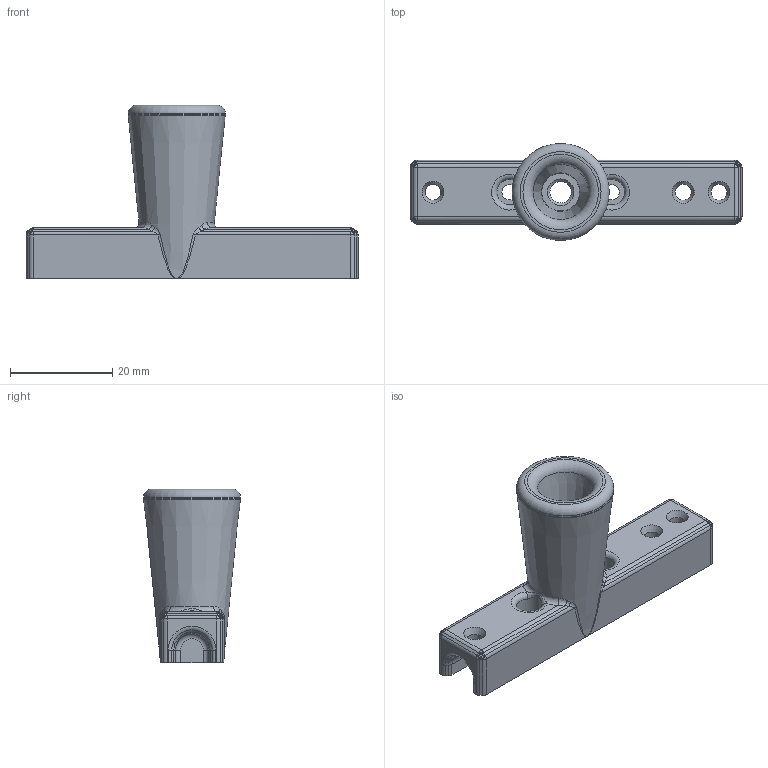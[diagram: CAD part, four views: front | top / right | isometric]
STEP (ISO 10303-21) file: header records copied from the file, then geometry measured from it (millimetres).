
FILE_DESCRIPTION(/* description */ (''),/* implementation_level */ '2;1');
FILE_NAME(/* name */ 'ARK Chargin'' Handle/UnfancyHandle/UnfawncyHandle.step',/* time_stamp */ '2022-02-03T00:25:49-07:00',/* author */ (''),/* organization */ (''),/* preprocessor_version */ 'ST-DEVELOPER v18.1',/* originating_system */ 'Autodesk Translation Framework v10.13.0.1454',/* authorisation */ '');
FILE_SCHEMA (('AUTOMOTIVE_DESIGN { 1 0 10303 214 3 1 1 }'));
Length unit declared in the file: millimetre
Products named in the file (1): UnfawncyHandle
Bounding box: 65 x 19 x 34 mm (x, y, z)
Volume: 10966.7 mm3; surface area: 5623.9 mm2
Topology: 1 solids, 1 shells, 175 faces, 398 edges, 222 vertices
Faces by surface type: cylinder 61, plane 45, sphere 24, bspline 22, cone 12, torus 11
Full cylindrical faces by diameter (mm): 3 x2, 3.1 x3, 4.2 x1, 5 x2, 7.4 x1, 19 x1
Entity records: 5592 total; most frequent: CARTESIAN_POINT 1678, DIRECTION 839, ORIENTED_EDGE 788, EDGE_CURVE 394, AXIS2_PLACEMENT_3D 332, VERTEX_POINT 222, EDGE_LOOP 188, FACE_OUTER_BOUND 175
